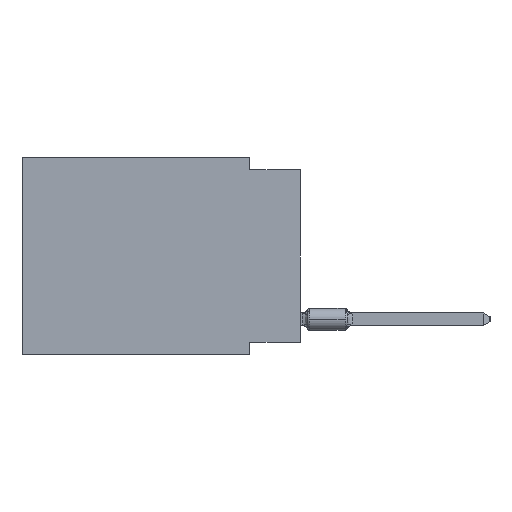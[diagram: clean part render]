
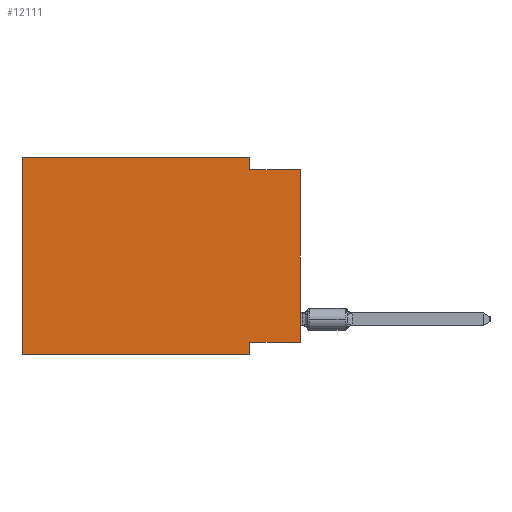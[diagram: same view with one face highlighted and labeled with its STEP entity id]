
A CAD part, left-side view. The second image highlights one B-rep face of the part: STEP entity #12111.
In plain terms, the highlighted planar face has unit normal (-1, 0, 0).
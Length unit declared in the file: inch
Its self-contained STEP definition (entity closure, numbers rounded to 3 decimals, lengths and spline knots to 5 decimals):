
#439 = ORIENTED_EDGE ( 'NONE', *, *, #461, .T. ) ;
#461 = EDGE_CURVE ( 'NONE', #14605, #26068, #2235, .T. ) ;
#2235 = LINE ( 'NONE', #9133, #40830 ) ;
#2662 = VECTOR ( 'NONE', #32391, 39.37008 ) ;
#3810 = EDGE_CURVE ( 'NONE', #16418, #27258, #13556, .T. ) ;
#4111 = LINE ( 'NONE', #26225, #30413 ) ;
#4320 = EDGE_CURVE ( 'NONE', #42305, #26068, #36999, .T. ) ;
#4661 = CARTESIAN_POINT ( 'NONE',  ( 0., 0.55, 0. ) ) ;
#5242 = CARTESIAN_POINT ( 'NONE',  ( 0., 0.1, -0.025 ) ) ;
#5530 = CARTESIAN_POINT ( 'NONE',  ( 0., 0.1, -0.39 ) ) ;
#6348 = CARTESIAN_POINT ( 'NONE',  ( 0., 0.1, -0.365 ) ) ;
#6741 = DIRECTION ( 'NONE',  ( 0., 1., 0. ) ) ;
#6822 = ORIENTED_EDGE ( 'NONE', *, *, #4320, .F. ) ;
#8800 = VECTOR ( 'NONE', #24266, 39.37008 ) ;
#8885 = ORIENTED_EDGE ( 'NONE', *, *, #3810, .F. ) ;
#9133 = CARTESIAN_POINT ( 'NONE',  ( 0., 0., 0. ) ) ;
#9134 = CARTESIAN_POINT ( 'NONE',  ( 0., 0.1, 0. ) ) ;
#9886 = CARTESIAN_POINT ( 'NONE',  ( 0., 0.55, -0.39 ) ) ;
#10690 = LINE ( 'NONE', #10922, #28153 ) ;
#10768 = CARTESIAN_POINT ( 'NONE',  ( 0., 0., -0.365 ) ) ;
#10922 = CARTESIAN_POINT ( 'NONE',  ( 0., 0.55, -0.39 ) ) ;
#11442 = ORIENTED_EDGE ( 'NONE', *, *, #30539, .F. ) ;
#12111 = ADVANCED_FACE ( 'NONE', ( #45862 ), #24442, .F. ) ;
#13271 = DIRECTION ( 'NONE',  ( 1., 0., 0. ) ) ;
#13556 = LINE ( 'NONE', #28069, #8800 ) ;
#13858 = LINE ( 'NONE', #27927, #26274 ) ;
#14199 = EDGE_CURVE ( 'NONE', #14605, #43765, #28614, .T. ) ;
#14331 = VECTOR ( 'NONE', #6741, 39.37008 ) ;
#14605 = VERTEX_POINT ( 'NONE', #32602 ) ;
#15272 = DIRECTION ( 'NONE',  ( 0., 0., -1. ) ) ;
#16418 = VERTEX_POINT ( 'NONE', #4661 ) ;
#16539 = ORIENTED_EDGE ( 'NONE', *, *, #30683, .T. ) ;
#17319 = CARTESIAN_POINT ( 'NONE',  ( 0., 0.55, 0. ) ) ;
#18173 = ORIENTED_EDGE ( 'NONE', *, *, #39245, .F. ) ;
#21204 = CARTESIAN_POINT ( 'NONE',  ( 0., 0.55, 0. ) ) ;
#22725 = DIRECTION ( 'NONE',  ( 0., -1., 0. ) ) ;
#22959 = CARTESIAN_POINT ( 'NONE',  ( 0., 0., -0.025 ) ) ;
#23961 = VERTEX_POINT ( 'NONE', #5530 ) ;
#24266 = DIRECTION ( 'NONE',  ( 0., -1., 0. ) ) ;
#24319 = LINE ( 'NONE', #21204, #2662 ) ;
#24442 = PLANE ( 'NONE',  #36836 ) ;
#26068 = VERTEX_POINT ( 'NONE', #26493 ) ;
#26225 = CARTESIAN_POINT ( 'NONE',  ( 0., 0.1, -0.39 ) ) ;
#26274 = VECTOR ( 'NONE', #35742, 39.37008 ) ;
#26493 = CARTESIAN_POINT ( 'NONE',  ( 0., 0., -0.025 ) ) ;
#26918 = VERTEX_POINT ( 'NONE', #9886 ) ;
#27258 = VERTEX_POINT ( 'NONE', #9134 ) ;
#27927 = CARTESIAN_POINT ( 'NONE',  ( 0., 0.1, 0. ) ) ;
#28069 = CARTESIAN_POINT ( 'NONE',  ( 0., 0.55, 0. ) ) ;
#28153 = VECTOR ( 'NONE', #43740, 39.37008 ) ;
#28614 = LINE ( 'NONE', #10768, #14331 ) ;
#30413 = VECTOR ( 'NONE', #15272, 39.37008 ) ;
#30539 = EDGE_CURVE ( 'NONE', #43765, #23961, #4111, .T. ) ;
#30683 = EDGE_CURVE ( 'NONE', #26918, #23961, #10690, .T. ) ;
#32391 = DIRECTION ( 'NONE',  ( 0., 0., 1. ) ) ;
#32602 = CARTESIAN_POINT ( 'NONE',  ( 0., 0., -0.365 ) ) ;
#35742 = DIRECTION ( 'NONE',  ( 0., 0., -1. ) ) ;
#36275 = ORIENTED_EDGE ( 'NONE', *, *, #38200, .F. ) ;
#36836 = AXIS2_PLACEMENT_3D ( 'NONE', #17319, #13271, #38488 ) ;
#36999 = LINE ( 'NONE', #22959, #42964 ) ;
#37447 = DIRECTION ( 'NONE',  ( 0., 0., 1. ) ) ;
#38200 = EDGE_CURVE ( 'NONE', #27258, #42305, #13858, .T. ) ;
#38488 = DIRECTION ( 'NONE',  ( 0., 0., -1. ) ) ;
#39245 = EDGE_CURVE ( 'NONE', #26918, #16418, #24319, .T. ) ;
#40536 = EDGE_LOOP ( 'NONE', ( #439, #6822, #36275, #8885, #18173, #16539, #11442, #43366 ) ) ;
#40830 = VECTOR ( 'NONE', #37447, 39.37008 ) ;
#42305 = VERTEX_POINT ( 'NONE', #5242 ) ;
#42964 = VECTOR ( 'NONE', #22725, 39.37008 ) ;
#43366 = ORIENTED_EDGE ( 'NONE', *, *, #14199, .F. ) ;
#43740 = DIRECTION ( 'NONE',  ( 0., -1., 0. ) ) ;
#43765 = VERTEX_POINT ( 'NONE', #6348 ) ;
#45862 = FACE_OUTER_BOUND ( 'NONE', #40536, .T. ) ;
